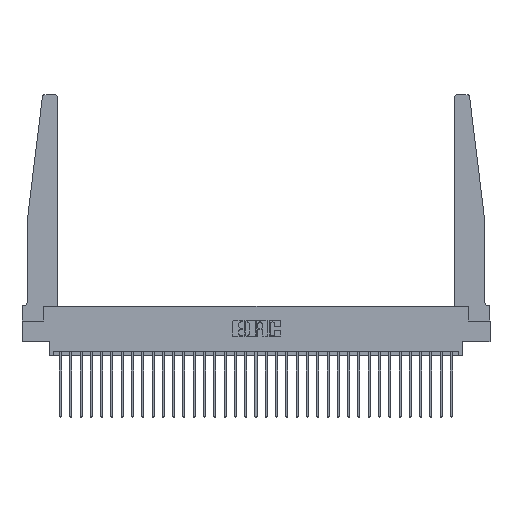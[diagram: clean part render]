
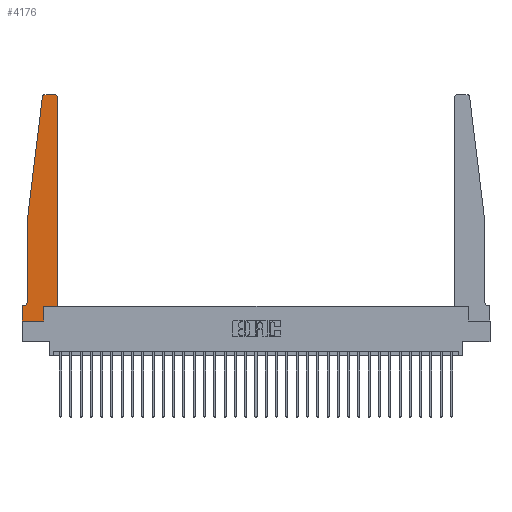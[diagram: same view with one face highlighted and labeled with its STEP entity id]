
A CAD part, top view. The second image highlights one B-rep face of the part: STEP entity #4176.
In plain terms, the highlighted planar face has unit normal (0, 0, 1).
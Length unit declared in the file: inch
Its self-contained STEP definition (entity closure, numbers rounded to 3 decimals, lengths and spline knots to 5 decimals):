
#11 = EDGE_CURVE ( 'NONE', #2073, #3396, #7940, .T. ) ;
#70 = DIRECTION ( 'NONE',  ( 0., -1., 0. ) ) ;
#143 = VERTEX_POINT ( 'NONE', #20977 ) ;
#261 = EDGE_CURVE ( 'NONE', #13072, #11405, #1169, .T. ) ;
#801 = VECTOR ( 'NONE', #29589, 39.37008 ) ;
#834 = CARTESIAN_POINT ( 'NONE',  ( 0.065, 0.2375, 0.37 ) ) ;
#1169 = LINE ( 'NONE', #23828, #25760 ) ;
#1312 = ORIENTED_EDGE ( 'NONE', *, *, #11, .T. ) ;
#1522 = AXIS2_PLACEMENT_3D ( 'NONE', #4745, #21410, #7151 ) ;
#1946 = LINE ( 'NONE', #7484, #19525 ) ;
#2073 = VERTEX_POINT ( 'NONE', #7719 ) ;
#2211 = LINE ( 'NONE', #19184, #7815 ) ;
#2333 = DIRECTION ( 'NONE',  ( 0., 0., 1. ) ) ;
#2633 = EDGE_CURVE ( 'NONE', #14157, #10347, #2211, .T. ) ;
#3396 = VERTEX_POINT ( 'NONE', #834 ) ;
#3742 = VERTEX_POINT ( 'NONE', #16670 ) ;
#4176 = ADVANCED_FACE ( 'NONE', ( #29995 ), #20537, .T. ) ;
#4429 = VERTEX_POINT ( 'NONE', #9393 ) ;
#4745 = CARTESIAN_POINT ( 'NONE',  ( 0.015, 0.2375, 0.37 ) ) ;
#6272 = CARTESIAN_POINT ( 'NONE',  ( 0., 0.1875, 0.37 ) ) ;
#7151 = DIRECTION ( 'NONE',  ( -1., 0., 0. ) ) ;
#7484 = CARTESIAN_POINT ( 'NONE',  ( 0.425, 0.18, 0.37 ) ) ;
#7719 = CARTESIAN_POINT ( 'NONE',  ( 0.065, 1.25, 0.37 ) ) ;
#7815 = VECTOR ( 'NONE', #12126, 39.37008 ) ;
#7940 = LINE ( 'NONE', #10671, #801 ) ;
#8304 = EDGE_CURVE ( 'NONE', #3396, #143, #12220, .T. ) ;
#8583 = AXIS2_PLACEMENT_3D ( 'NONE', #6272, #13483, #30012 ) ;
#8933 = CARTESIAN_POINT ( 'NONE',  ( 0.2605, 0.18, 0.37 ) ) ;
#9257 = AXIS2_PLACEMENT_3D ( 'NONE', #13595, #30110, #16005 ) ;
#9393 = CARTESIAN_POINT ( 'NONE',  ( 0.425, 0.18, 0.37 ) ) ;
#9917 = VECTOR ( 'NONE', #29784, 39.37008 ) ;
#10347 = VERTEX_POINT ( 'NONE', #20456 ) ;
#10379 = VECTOR ( 'NONE', #14958, 39.37008 ) ;
#10671 = CARTESIAN_POINT ( 'NONE',  ( 0.065, 1.25, 0.37 ) ) ;
#10679 = CIRCLE ( 'NONE', #26202, 0.03 ) ;
#10692 = EDGE_CURVE ( 'NONE', #11426, #14799, #15044, .T. ) ;
#10855 = CARTESIAN_POINT ( 'NONE',  ( 0.425, 0.18, 0.37 ) ) ;
#11405 = VERTEX_POINT ( 'NONE', #30645 ) ;
#11426 = VERTEX_POINT ( 'NONE', #14116 ) ;
#11793 = EDGE_LOOP ( 'NONE', ( #18893, #19622, #14066, #1312, #18179, #22198, #30724, #22932, #11838, #27393, #17249, #17304 ) ) ;
#11838 = ORIENTED_EDGE ( 'NONE', *, *, #10692, .T. ) ;
#12126 = DIRECTION ( 'NONE',  ( -1., 0., 0. ) ) ;
#12220 = CIRCLE ( 'NONE', #1522, 0.05 ) ;
#12338 = VECTOR ( 'NONE', #22131, 39.37008 ) ;
#12451 = EDGE_CURVE ( 'NONE', #143, #13072, #13821, .T. ) ;
#13072 = VERTEX_POINT ( 'NONE', #13403 ) ;
#13312 = EDGE_CURVE ( 'NONE', #10347, #20458, #14508, .T. ) ;
#13375 = CARTESIAN_POINT ( 'NONE',  ( 0.065, 1.25, 0.37 ) ) ;
#13403 = CARTESIAN_POINT ( 'NONE',  ( 0., 0.1875, 0.37 ) ) ;
#13483 = DIRECTION ( 'NONE',  ( 0., 0., 1. ) ) ;
#13595 = CARTESIAN_POINT ( 'NONE',  ( 0.27653, 2.72, 0.37 ) ) ;
#13821 = LINE ( 'NONE', #15096, #12338 ) ;
#14066 = ORIENTED_EDGE ( 'NONE', *, *, #19097, .T. ) ;
#14116 = CARTESIAN_POINT ( 'NONE',  ( 0.2605, 0., 0.37 ) ) ;
#14157 = VERTEX_POINT ( 'NONE', #30595 ) ;
#14508 = CIRCLE ( 'NONE', #9257, 0.03 ) ;
#14799 = VERTEX_POINT ( 'NONE', #27992 ) ;
#14958 = DIRECTION ( 'NONE',  ( 1., 0., 0. ) ) ;
#15044 = LINE ( 'NONE', #8933, #24639 ) ;
#15096 = CARTESIAN_POINT ( 'NONE',  ( 0.065, 0.1875, 0.37 ) ) ;
#15971 = EDGE_CURVE ( 'NONE', #3742, #14157, #10679, .T. ) ;
#16005 = DIRECTION ( 'NONE',  ( 1., 0., 0. ) ) ;
#16670 = CARTESIAN_POINT ( 'NONE',  ( 0.425, 2.72, 0.37 ) ) ;
#16703 = CARTESIAN_POINT ( 'NONE',  ( 0.395, 2.72, 0.37 ) ) ;
#17249 = ORIENTED_EDGE ( 'NONE', *, *, #20225, .T. ) ;
#17304 = ORIENTED_EDGE ( 'NONE', *, *, #15971, .T. ) ;
#18179 = ORIENTED_EDGE ( 'NONE', *, *, #8304, .T. ) ;
#18668 = CARTESIAN_POINT ( 'NONE',  ( 0.24675, 2.72367, 0.37 ) ) ;
#18893 = ORIENTED_EDGE ( 'NONE', *, *, #2633, .T. ) ;
#19061 = DIRECTION ( 'NONE',  ( 1., 0., 0. ) ) ;
#19097 = EDGE_CURVE ( 'NONE', #20458, #2073, #23890, .T. ) ;
#19184 = CARTESIAN_POINT ( 'NONE',  ( 0.25, 2.75, 0.37 ) ) ;
#19525 = VECTOR ( 'NONE', #21861, 39.37008 ) ;
#19622 = ORIENTED_EDGE ( 'NONE', *, *, #13312, .T. ) ;
#20225 = EDGE_CURVE ( 'NONE', #4429, #3742, #30290, .T. ) ;
#20456 = CARTESIAN_POINT ( 'NONE',  ( 0.27653, 2.75, 0.37 ) ) ;
#20458 = VERTEX_POINT ( 'NONE', #18668 ) ;
#20537 = PLANE ( 'NONE',  #8583 ) ;
#20800 = DIRECTION ( 'NONE',  ( 0., 1., 0. ) ) ;
#20977 = CARTESIAN_POINT ( 'NONE',  ( 0.015, 0.1875, 0.37 ) ) ;
#21410 = DIRECTION ( 'NONE',  ( 0., 0., -1. ) ) ;
#21861 = DIRECTION ( 'NONE',  ( 1., 0., 0. ) ) ;
#22131 = DIRECTION ( 'NONE',  ( -1., 0., 0. ) ) ;
#22198 = ORIENTED_EDGE ( 'NONE', *, *, #12451, .T. ) ;
#22932 = ORIENTED_EDGE ( 'NONE', *, *, #30549, .T. ) ;
#23013 = LINE ( 'NONE', #24346, #10379 ) ;
#23828 = CARTESIAN_POINT ( 'NONE',  ( 0., 0., 0.37 ) ) ;
#23890 = LINE ( 'NONE', #13375, #29402 ) ;
#24346 = CARTESIAN_POINT ( 'NONE',  ( 0., 0., 0.37 ) ) ;
#24639 = VECTOR ( 'NONE', #20800, 39.37008 ) ;
#25251 = DIRECTION ( 'NONE',  ( -0.122, -0.992, 0. ) ) ;
#25760 = VECTOR ( 'NONE', #70, 39.37008 ) ;
#26202 = AXIS2_PLACEMENT_3D ( 'NONE', #16703, #2333, #19061 ) ;
#27393 = ORIENTED_EDGE ( 'NONE', *, *, #27762, .T. ) ;
#27762 = EDGE_CURVE ( 'NONE', #14799, #4429, #1946, .T. ) ;
#27992 = CARTESIAN_POINT ( 'NONE',  ( 0.2605, 0.18, 0.37 ) ) ;
#29402 = VECTOR ( 'NONE', #25251, 39.37008 ) ;
#29589 = DIRECTION ( 'NONE',  ( 0., -1., 0. ) ) ;
#29784 = DIRECTION ( 'NONE',  ( 0., 1., 0. ) ) ;
#29995 = FACE_OUTER_BOUND ( 'NONE', #11793, .T. ) ;
#30012 = DIRECTION ( 'NONE',  ( 1., 0., 0. ) ) ;
#30110 = DIRECTION ( 'NONE',  ( 0., 0., 1. ) ) ;
#30290 = LINE ( 'NONE', #10855, #9917 ) ;
#30549 = EDGE_CURVE ( 'NONE', #11405, #11426, #23013, .T. ) ;
#30595 = CARTESIAN_POINT ( 'NONE',  ( 0.395, 2.75, 0.37 ) ) ;
#30645 = CARTESIAN_POINT ( 'NONE',  ( 0., 0., 0.37 ) ) ;
#30724 = ORIENTED_EDGE ( 'NONE', *, *, #261, .T. ) ;
